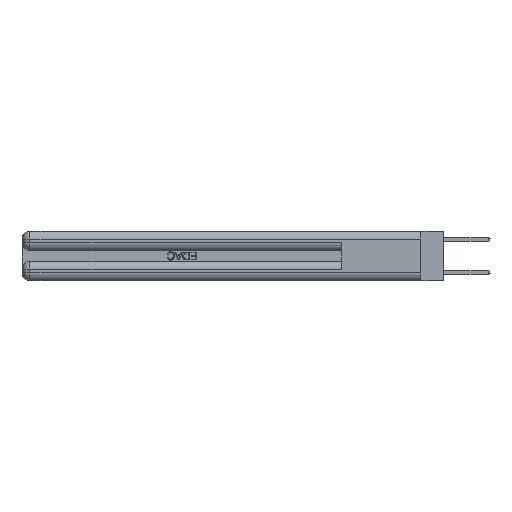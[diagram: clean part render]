
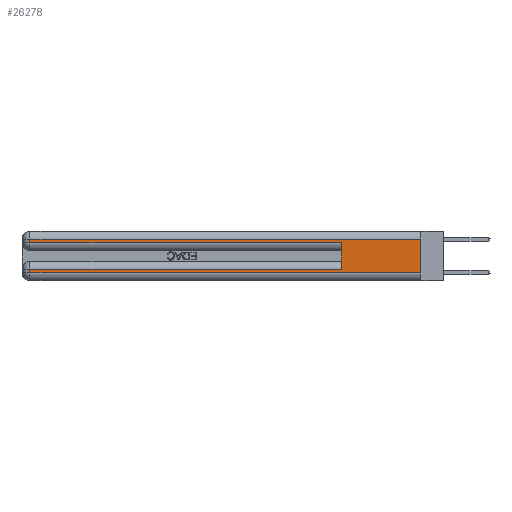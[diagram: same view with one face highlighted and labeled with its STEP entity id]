
A CAD part, left-side view. The second image highlights one B-rep face of the part: STEP entity #26278.
In plain terms, the highlighted planar face has unit normal (-1, 0, 0).
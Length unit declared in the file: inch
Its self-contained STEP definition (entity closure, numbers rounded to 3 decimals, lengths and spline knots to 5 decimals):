
#398 = VECTOR ( 'NONE', #5972, 39.37008 ) ;
#519 = LINE ( 'NONE', #16108, #11146 ) ;
#583 = LINE ( 'NONE', #736, #11159 ) ;
#736 = CARTESIAN_POINT ( 'NONE',  ( 0., 0.6, 0.145 ) ) ;
#1787 = EDGE_CURVE ( 'NONE', #4153, #21588, #583, .T. ) ;
#3024 = CARTESIAN_POINT ( 'NONE',  ( 0., 0., 0.31 ) ) ;
#3657 = DIRECTION ( 'NONE',  ( 0., 0., -1. ) ) ;
#4153 = VERTEX_POINT ( 'NONE', #9179 ) ;
#5039 = VECTOR ( 'NONE', #11322, 39.37008 ) ;
#5044 = EDGE_CURVE ( 'NONE', #15862, #21588, #20600, .T. ) ;
#5171 = VECTOR ( 'NONE', #3657, 39.37008 ) ;
#5366 = CARTESIAN_POINT ( 'NONE',  ( 0., 2.94, 0.06 ) ) ;
#5972 = DIRECTION ( 'NONE',  ( 0., 0., -1. ) ) ;
#6023 = VECTOR ( 'NONE', #20529, 39.37008 ) ;
#6636 = ORIENTED_EDGE ( 'NONE', *, *, #22118, .T. ) ;
#6942 = CARTESIAN_POINT ( 'NONE',  ( 0., 0., 0.37 ) ) ;
#7005 = FACE_OUTER_BOUND ( 'NONE', #25096, .T. ) ;
#8289 = EDGE_CURVE ( 'NONE', #22532, #8980, #519, .T. ) ;
#8980 = VERTEX_POINT ( 'NONE', #10600 ) ;
#9179 = CARTESIAN_POINT ( 'NONE',  ( 0., 0.6, 0.085 ) ) ;
#9655 = DIRECTION ( 'NONE',  ( 1., 0., 0. ) ) ;
#10600 = CARTESIAN_POINT ( 'NONE',  ( 0., 0., 0.06 ) ) ;
#10769 = EDGE_CURVE ( 'NONE', #28353, #15862, #17196, .T. ) ;
#11146 = VECTOR ( 'NONE', #18624, 39.37008 ) ;
#11159 = VECTOR ( 'NONE', #11755, 39.37008 ) ;
#11231 = CARTESIAN_POINT ( 'NONE',  ( 0., 0., 0.085 ) ) ;
#11322 = DIRECTION ( 'NONE',  ( 0., -1., 0. ) ) ;
#11363 = ORIENTED_EDGE ( 'NONE', *, *, #5044, .T. ) ;
#11696 = CARTESIAN_POINT ( 'NONE',  ( 0., 0., 0.31 ) ) ;
#11755 = DIRECTION ( 'NONE',  ( 0., 0., 1. ) ) ;
#12313 = ORIENTED_EDGE ( 'NONE', *, *, #19826, .F. ) ;
#12785 = ORIENTED_EDGE ( 'NONE', *, *, #10769, .T. ) ;
#13077 = CARTESIAN_POINT ( 'NONE',  ( 0., 2.94, 0.285 ) ) ;
#15036 = AXIS2_PLACEMENT_3D ( 'NONE', #16148, #9655, #20709 ) ;
#15074 = DIRECTION ( 'NONE',  ( 0., 1., 0. ) ) ;
#15122 = CARTESIAN_POINT ( 'NONE',  ( 0., 2.94, 0.37 ) ) ;
#15862 = VERTEX_POINT ( 'NONE', #13077 ) ;
#15944 = DIRECTION ( 'NONE',  ( 0., 0., -1. ) ) ;
#16108 = CARTESIAN_POINT ( 'NONE',  ( 0., 0., 0.06 ) ) ;
#16148 = CARTESIAN_POINT ( 'NONE',  ( 0., 0., 0.37 ) ) ;
#16581 = CARTESIAN_POINT ( 'NONE',  ( 0., 2.94, 0.37 ) ) ;
#16839 = VECTOR ( 'NONE', #15074, 39.37008 ) ;
#17111 = VERTEX_POINT ( 'NONE', #27691 ) ;
#17196 = LINE ( 'NONE', #15122, #5171 ) ;
#17515 = CARTESIAN_POINT ( 'NONE',  ( 0., 0.6, 0.285 ) ) ;
#17588 = LINE ( 'NONE', #11231, #16839 ) ;
#18624 = DIRECTION ( 'NONE',  ( 0., -1., 0. ) ) ;
#19077 = VECTOR ( 'NONE', #15944, 39.37008 ) ;
#19826 = EDGE_CURVE ( 'NONE', #25697, #8980, #27277, .T. ) ;
#20529 = DIRECTION ( 'NONE',  ( 0., 1., 0. ) ) ;
#20600 = LINE ( 'NONE', #20742, #5039 ) ;
#20709 = DIRECTION ( 'NONE',  ( 0., 0., -1. ) ) ;
#20742 = CARTESIAN_POINT ( 'NONE',  ( 0., 0., 0.285 ) ) ;
#20765 = ORIENTED_EDGE ( 'NONE', *, *, #1787, .F. ) ;
#21588 = VERTEX_POINT ( 'NONE', #17515 ) ;
#22118 = EDGE_CURVE ( 'NONE', #17111, #22532, #23604, .T. ) ;
#22314 = EDGE_CURVE ( 'NONE', #25697, #28353, #24934, .T. ) ;
#22344 = ORIENTED_EDGE ( 'NONE', *, *, #22314, .T. ) ;
#22532 = VERTEX_POINT ( 'NONE', #5366 ) ;
#23604 = LINE ( 'NONE', #16581, #398 ) ;
#24099 = EDGE_CURVE ( 'NONE', #4153, #17111, #17588, .T. ) ;
#24934 = LINE ( 'NONE', #11696, #6023 ) ;
#25096 = EDGE_LOOP ( 'NONE', ( #12313, #22344, #12785, #11363, #20765, #27457, #6636, #27298 ) ) ;
#25697 = VERTEX_POINT ( 'NONE', #3024 ) ;
#26278 = ADVANCED_FACE ( 'NONE', ( #7005 ), #27480, .F. ) ;
#26799 = CARTESIAN_POINT ( 'NONE',  ( 0., 2.94, 0.31 ) ) ;
#27277 = LINE ( 'NONE', #6942, #19077 ) ;
#27298 = ORIENTED_EDGE ( 'NONE', *, *, #8289, .T. ) ;
#27457 = ORIENTED_EDGE ( 'NONE', *, *, #24099, .T. ) ;
#27480 = PLANE ( 'NONE',  #15036 ) ;
#27691 = CARTESIAN_POINT ( 'NONE',  ( 0., 2.94, 0.085 ) ) ;
#28353 = VERTEX_POINT ( 'NONE', #26799 ) ;
